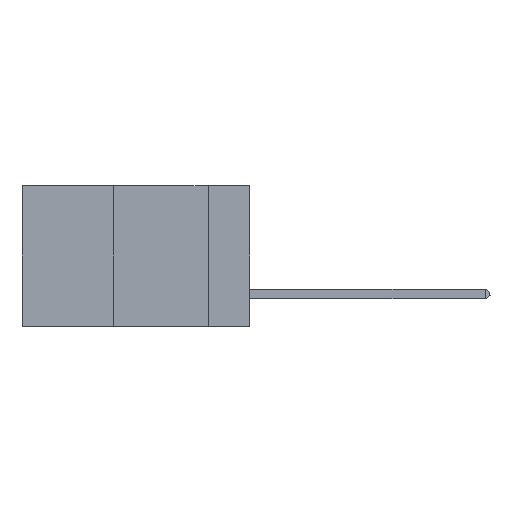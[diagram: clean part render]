
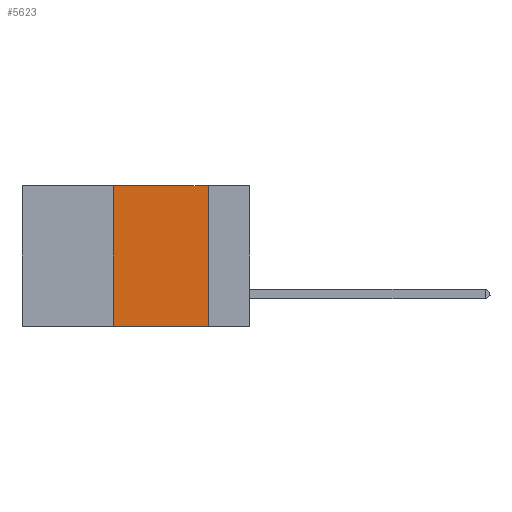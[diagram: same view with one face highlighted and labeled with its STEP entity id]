
A CAD part, left-side view. The second image highlights one B-rep face of the part: STEP entity #5623.
In plain terms, the highlighted planar face has unit normal (-1, 0, 0).
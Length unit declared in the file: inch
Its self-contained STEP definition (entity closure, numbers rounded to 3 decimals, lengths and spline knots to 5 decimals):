
#286 = ORIENTED_EDGE ( 'NONE', *, *, #2643, .F. ) ;
#339 = VERTEX_POINT ( 'NONE', #3568 ) ;
#642 = DIRECTION ( 'NONE',  ( 0., 0., -1. ) ) ;
#1043 = EDGE_CURVE ( 'NONE', #12086, #5554, #2332, .T. ) ;
#1707 = CARTESIAN_POINT ( 'NONE',  ( 0., 0.36, -0.37 ) ) ;
#2332 = LINE ( 'NONE', #5644, #11147 ) ;
#2643 = EDGE_CURVE ( 'NONE', #8430, #339, #9104, .T. ) ;
#3568 = CARTESIAN_POINT ( 'NONE',  ( 0., 0.11, 0. ) ) ;
#3602 = ORIENTED_EDGE ( 'NONE', *, *, #4343, .F. ) ;
#3716 = CARTESIAN_POINT ( 'NONE',  ( 0., 0.11, 0. ) ) ;
#3898 = CARTESIAN_POINT ( 'NONE',  ( 0., 0.36, 0. ) ) ;
#4237 = ORIENTED_EDGE ( 'NONE', *, *, #6426, .F. ) ;
#4343 = EDGE_CURVE ( 'NONE', #12086, #8430, #7093, .T. ) ;
#5554 = VERTEX_POINT ( 'NONE', #6268 ) ;
#5623 = ADVANCED_FACE ( 'NONE', ( #6013 ), #8554, .F. ) ;
#5644 = CARTESIAN_POINT ( 'NONE',  ( 0., 0.6, -0.37 ) ) ;
#6013 = FACE_OUTER_BOUND ( 'NONE', #11783, .T. ) ;
#6268 = CARTESIAN_POINT ( 'NONE',  ( 0., 0.11, -0.37 ) ) ;
#6426 = EDGE_CURVE ( 'NONE', #339, #5554, #6922, .T. ) ;
#6491 = DIRECTION ( 'NONE',  ( 1., 0., 0. ) ) ;
#6922 = LINE ( 'NONE', #3716, #7077 ) ;
#7077 = VECTOR ( 'NONE', #11454, 39.37008 ) ;
#7093 = LINE ( 'NONE', #3898, #12264 ) ;
#7422 = CARTESIAN_POINT ( 'NONE',  ( 0., 0.36, 0. ) ) ;
#7428 = VECTOR ( 'NONE', #8025, 39.37008 ) ;
#7541 = DIRECTION ( 'NONE',  ( 0., -1., 0. ) ) ;
#8025 = DIRECTION ( 'NONE',  ( 0., -1., 0. ) ) ;
#8430 = VERTEX_POINT ( 'NONE', #7422 ) ;
#8554 = PLANE ( 'NONE',  #9125 ) ;
#9104 = LINE ( 'NONE', #10285, #7428 ) ;
#9125 = AXIS2_PLACEMENT_3D ( 'NONE', #12295, #6491, #642 ) ;
#10079 = ORIENTED_EDGE ( 'NONE', *, *, #1043, .T. ) ;
#10285 = CARTESIAN_POINT ( 'NONE',  ( 0., 0.6, 0. ) ) ;
#11147 = VECTOR ( 'NONE', #7541, 39.37008 ) ;
#11454 = DIRECTION ( 'NONE',  ( 0., 0., -1. ) ) ;
#11688 = DIRECTION ( 'NONE',  ( 0., 0., 1. ) ) ;
#11783 = EDGE_LOOP ( 'NONE', ( #4237, #286, #3602, #10079 ) ) ;
#12086 = VERTEX_POINT ( 'NONE', #1707 ) ;
#12264 = VECTOR ( 'NONE', #11688, 39.37008 ) ;
#12295 = CARTESIAN_POINT ( 'NONE',  ( 0., 0.6, 0. ) ) ;
